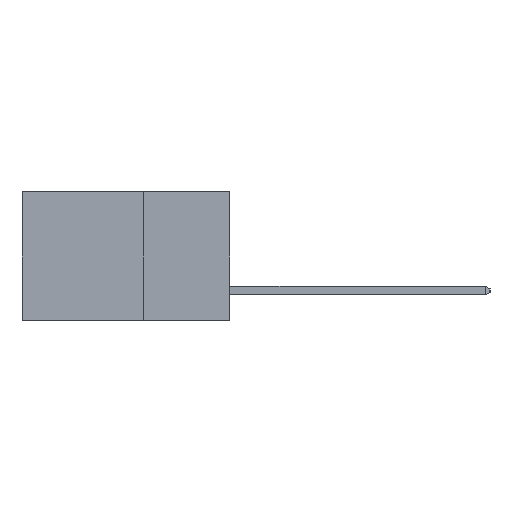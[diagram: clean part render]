
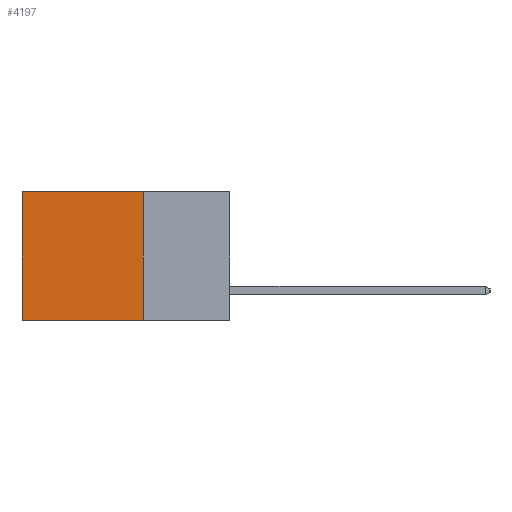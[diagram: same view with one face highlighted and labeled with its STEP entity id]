
A CAD part, left-side view. The second image highlights one B-rep face of the part: STEP entity #4197.
In plain terms, the highlighted planar face has unit normal (-1, 0, 0).
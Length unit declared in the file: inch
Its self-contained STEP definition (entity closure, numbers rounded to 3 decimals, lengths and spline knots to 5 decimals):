
#2 = EDGE_LOOP ( 'NONE', ( #4091, #11458, #13833, #1929 ) ) ;
#341 = DIRECTION ( 'NONE',  ( 0., 1., 0. ) ) ;
#745 = CARTESIAN_POINT ( 'NONE',  ( 0.2615, 0.25, -0.37 ) ) ;
#749 = VERTEX_POINT ( 'NONE', #745 ) ;
#980 = CARTESIAN_POINT ( 'NONE',  ( 0.2615, 0.25, 0. ) ) ;
#1146 = DIRECTION ( 'NONE',  ( 0., 0., -1. ) ) ;
#1929 = ORIENTED_EDGE ( 'NONE', *, *, #10802, .T. ) ;
#2065 = CARTESIAN_POINT ( 'NONE',  ( 0.2615, 0.25, -0.37 ) ) ;
#2258 = LINE ( 'NONE', #8029, #8367 ) ;
#2669 = VERTEX_POINT ( 'NONE', #980 ) ;
#2884 = LINE ( 'NONE', #11478, #14302 ) ;
#3338 = VERTEX_POINT ( 'NONE', #7992 ) ;
#3753 = VECTOR ( 'NONE', #10008, 39.37008 ) ;
#4091 = ORIENTED_EDGE ( 'NONE', *, *, #13458, .T. ) ;
#4197 = ADVANCED_FACE ( 'NONE', ( #9833 ), #7871, .F. ) ;
#6090 = CARTESIAN_POINT ( 'NONE',  ( 0.2615, 0.25, -0.37 ) ) ;
#6201 = AXIS2_PLACEMENT_3D ( 'NONE', #8149, #7806, #7755 ) ;
#6765 = CARTESIAN_POINT ( 'NONE',  ( 0.2615, 0.6, -0.37 ) ) ;
#7755 = DIRECTION ( 'NONE',  ( 0., 0., -1. ) ) ;
#7806 = DIRECTION ( 'NONE',  ( 1., 0., 0. ) ) ;
#7871 = PLANE ( 'NONE',  #6201 ) ;
#7992 = CARTESIAN_POINT ( 'NONE',  ( 0.2615, 0.6, 0. ) ) ;
#8029 = CARTESIAN_POINT ( 'NONE',  ( 0.2615, 0.6, -0.37 ) ) ;
#8149 = CARTESIAN_POINT ( 'NONE',  ( 0.2615, 0.25, -0.37 ) ) ;
#8367 = VECTOR ( 'NONE', #1146, 39.37008 ) ;
#8868 = LINE ( 'NONE', #6090, #11093 ) ;
#9833 = FACE_OUTER_BOUND ( 'NONE', #2, .T. ) ;
#10008 = DIRECTION ( 'NONE',  ( 0., 0., -1. ) ) ;
#10458 = DIRECTION ( 'NONE',  ( 0., 1., 0. ) ) ;
#10618 = VERTEX_POINT ( 'NONE', #6765 ) ;
#10802 = EDGE_CURVE ( 'NONE', #2669, #3338, #2884, .T. ) ;
#11093 = VECTOR ( 'NONE', #341, 39.37008 ) ;
#11458 = ORIENTED_EDGE ( 'NONE', *, *, #13675, .F. ) ;
#11478 = CARTESIAN_POINT ( 'NONE',  ( 0.2615, 0.25, 0. ) ) ;
#12238 = LINE ( 'NONE', #2065, #3753 ) ;
#13458 = EDGE_CURVE ( 'NONE', #3338, #10618, #2258, .T. ) ;
#13675 = EDGE_CURVE ( 'NONE', #749, #10618, #8868, .T. ) ;
#13833 = ORIENTED_EDGE ( 'NONE', *, *, #13980, .F. ) ;
#13980 = EDGE_CURVE ( 'NONE', #2669, #749, #12238, .T. ) ;
#14302 = VECTOR ( 'NONE', #10458, 39.37008 ) ;
